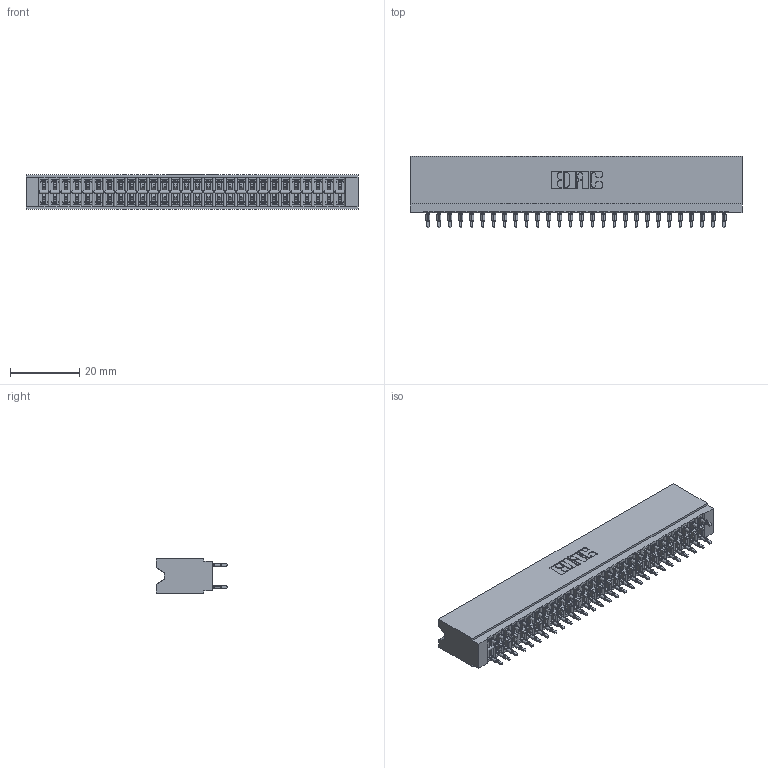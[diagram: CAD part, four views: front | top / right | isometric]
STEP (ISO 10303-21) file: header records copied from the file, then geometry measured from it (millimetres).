
FILE_DESCRIPTION (( 'STEP AP203' ), '1' );
FILE_NAME ('746-056-560-206.STEP', '2026-02-27T19:55:42', ( '' ), ( '' ), 'SwSTEP 2.0', 'SolidWorks 2023', '' );
FILE_SCHEMA (( 'CONFIG_CONTROL_DESIGN' ));
Length unit declared in the file: millimetre
Products named in the file (3): 746-056-560-206; 746 Part_.515 Slot Depth - 06; 746-292-001_560
Assembly tree (57 placements, depth 2):
  746-056-560-206
    746 Part_.515 Slot Depth - 06
    746-292-001_560  x56
Bounding box: 96.14 x 20.82 x 9.91 mm (x, y, z)
Volume: 10566.2 mm3; surface area: 17617.2 mm2
Topology: 57 solids, 57 shells, 5390 faces, 14993 edges, 9611 vertices
Faces by surface type: plane 2688, cylinder 1246, bspline 1120, torus 336
Entity records: 45392 total; most frequent: CARTESIAN_POINT 9142, ORIENTED_EDGE 7766, DIRECTION 6515, EDGE_CURVE 3883, VECTOR 3411, LINE 3411, VERTEX_POINT 2571, AXIS2_PLACEMENT_3D 1552
